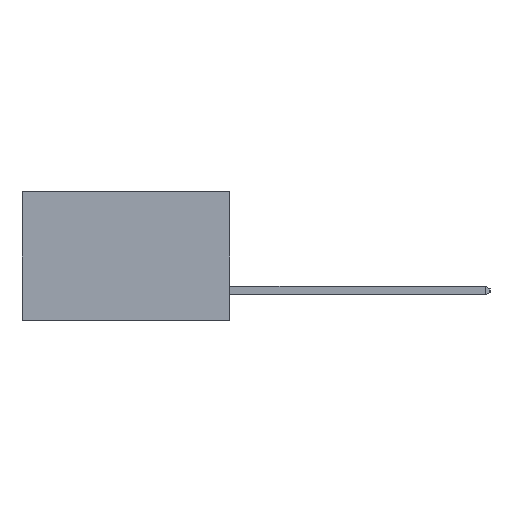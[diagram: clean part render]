
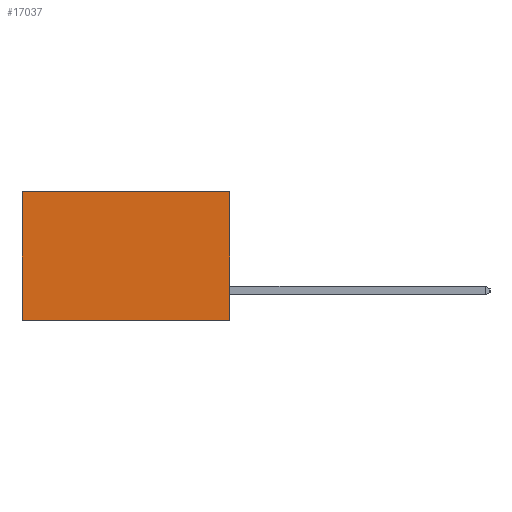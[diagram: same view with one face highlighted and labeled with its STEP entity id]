
A CAD part, left-side view. The second image highlights one B-rep face of the part: STEP entity #17037.
In plain terms, the highlighted planar face has unit normal (-1, 0, 0).
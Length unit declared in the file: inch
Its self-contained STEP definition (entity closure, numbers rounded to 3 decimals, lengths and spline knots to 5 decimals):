
#260 = ORIENTED_EDGE ( 'NONE', *, *, #814, .T. ) ;
#375 = VECTOR ( 'NONE', #15334, 39.37008 ) ;
#787 = FACE_OUTER_BOUND ( 'NONE', #8399, .T. ) ;
#814 = EDGE_CURVE ( 'NONE', #20542, #1222, #13802, .T. ) ;
#1222 = VERTEX_POINT ( 'NONE', #7133 ) ;
#1940 = VECTOR ( 'NONE', #10794, 39.37008 ) ;
#2994 = CARTESIAN_POINT ( 'NONE',  ( 0.2615, 0., -0.37 ) ) ;
#3103 = DIRECTION ( 'NONE',  ( 0., 0., -1. ) ) ;
#4043 = DIRECTION ( 'NONE',  ( 0., 0., -1. ) ) ;
#4109 = DIRECTION ( 'NONE',  ( 1., 0., 0. ) ) ;
#4249 = PLANE ( 'NONE',  #10739 ) ;
#4668 = CARTESIAN_POINT ( 'NONE',  ( 0.2615, 0., -0.37 ) ) ;
#6027 = VECTOR ( 'NONE', #3103, 39.37008 ) ;
#7133 = CARTESIAN_POINT ( 'NONE',  ( 0.2615, 0.6, -0.37 ) ) ;
#7325 = DIRECTION ( 'NONE',  ( 0., 1., 0. ) ) ;
#7474 = CARTESIAN_POINT ( 'NONE',  ( 0.2615, 0., -0.37 ) ) ;
#8319 = EDGE_CURVE ( 'NONE', #14105, #13194, #19331, .T. ) ;
#8399 = EDGE_LOOP ( 'NONE', ( #260, #17743, #11235, #14022 ) ) ;
#9124 = CARTESIAN_POINT ( 'NONE',  ( 0.2615, 0., 0. ) ) ;
#9741 = CARTESIAN_POINT ( 'NONE',  ( 0.2615, 0.6, -0.37 ) ) ;
#10739 = AXIS2_PLACEMENT_3D ( 'NONE', #4668, #4109, #4043 ) ;
#10794 = DIRECTION ( 'NONE',  ( 0., 1., 0. ) ) ;
#11235 = ORIENTED_EDGE ( 'NONE', *, *, #8319, .F. ) ;
#12037 = CARTESIAN_POINT ( 'NONE',  ( 0.2615, 0.6, 0. ) ) ;
#12323 = EDGE_CURVE ( 'NONE', #13194, #1222, #18837, .T. ) ;
#13194 = VERTEX_POINT ( 'NONE', #14083 ) ;
#13802 = LINE ( 'NONE', #9741, #375 ) ;
#14022 = ORIENTED_EDGE ( 'NONE', *, *, #20711, .T. ) ;
#14083 = CARTESIAN_POINT ( 'NONE',  ( 0.2615, 0., -0.37 ) ) ;
#14105 = VERTEX_POINT ( 'NONE', #20734 ) ;
#14480 = VECTOR ( 'NONE', #7325, 39.37008 ) ;
#15334 = DIRECTION ( 'NONE',  ( 0., 0., -1. ) ) ;
#17037 = ADVANCED_FACE ( 'NONE', ( #787 ), #4249, .F. ) ;
#17743 = ORIENTED_EDGE ( 'NONE', *, *, #12323, .F. ) ;
#18837 = LINE ( 'NONE', #7474, #14480 ) ;
#19331 = LINE ( 'NONE', #2994, #6027 ) ;
#20163 = LINE ( 'NONE', #9124, #1940 ) ;
#20542 = VERTEX_POINT ( 'NONE', #12037 ) ;
#20711 = EDGE_CURVE ( 'NONE', #14105, #20542, #20163, .T. ) ;
#20734 = CARTESIAN_POINT ( 'NONE',  ( 0.2615, 0., 0. ) ) ;
